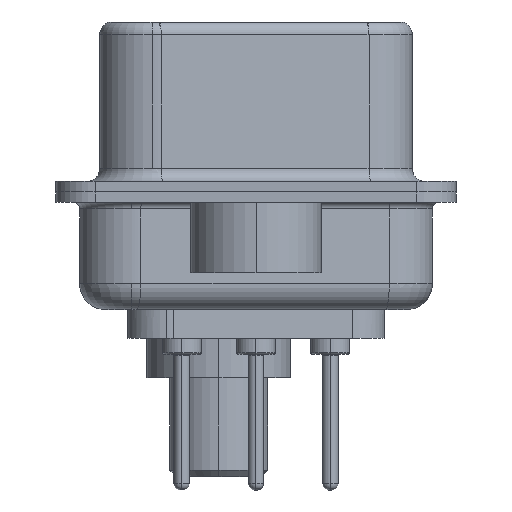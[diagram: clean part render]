
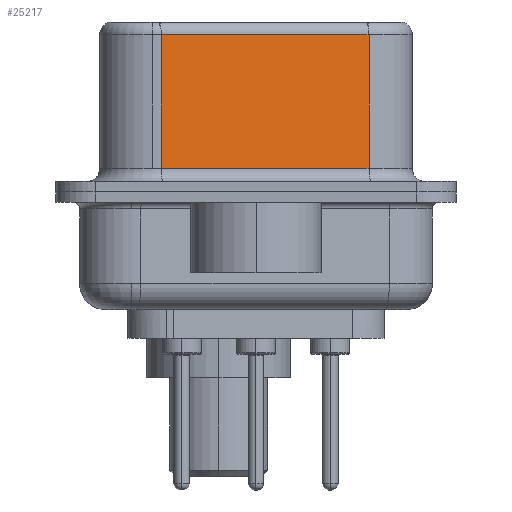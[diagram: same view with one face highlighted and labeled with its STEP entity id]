
A CAD part, left-side view. The second image highlights one B-rep face of the part: STEP entity #25217.
In plain terms, the highlighted planar face has unit normal (-0.985, -0.174, 0).
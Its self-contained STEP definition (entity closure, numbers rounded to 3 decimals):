
#1326 = AXIS2_PLACEMENT_3D ( 'NONE', #9532, #11748, #26969 ) ;
#1716 = VERTEX_POINT ( 'NONE', #25564 ) ;
#1884 = CARTESIAN_POINT ( 'NONE',  ( 3.73, 3.628, 6.52 ) ) ;
#2103 = EDGE_CURVE ( 'NONE', #10465, #1716, #22471, .T. ) ;
#4481 = CARTESIAN_POINT ( 'NONE',  ( 5.132, -4.322, 0.9 ) ) ;
#7355 = PLANE ( 'NONE',  #1326 ) ;
#7525 = LINE ( 'NONE', #1884, #24196 ) ;
#8537 = EDGE_CURVE ( 'NONE', #21673, #17644, #7525, .T. ) ;
#9532 = CARTESIAN_POINT ( 'NONE',  ( 5.132, -4.322, 6.52 ) ) ;
#10465 = VERTEX_POINT ( 'NONE', #26105 ) ;
#10806 = DIRECTION ( 'NONE',  ( 0., 0., -1. ) ) ;
#11016 = DIRECTION ( 'NONE',  ( 0.174, -0.985, 0. ) ) ;
#11748 = DIRECTION ( 'NONE',  ( 0.985, 0.174, 0. ) ) ;
#12886 = ORIENTED_EDGE ( 'NONE', *, *, #16227, .T. ) ;
#13771 = LINE ( 'NONE', #4481, #16933 ) ;
#14318 = CARTESIAN_POINT ( 'NONE',  ( 5.132, -4.322, 6.02 ) ) ;
#14321 = CARTESIAN_POINT ( 'NONE',  ( 5.132, -4.322, 6.52 ) ) ;
#15447 = DIRECTION ( 'NONE',  ( 0., 0., -1. ) ) ;
#16227 = EDGE_CURVE ( 'NONE', #17644, #1716, #13771, .T. ) ;
#16933 = VECTOR ( 'NONE', #11016, 1000. ) ;
#17644 = VERTEX_POINT ( 'NONE', #19032 ) ;
#18451 = CARTESIAN_POINT ( 'NONE',  ( 3.73, 3.628, 6.02 ) ) ;
#19032 = CARTESIAN_POINT ( 'NONE',  ( 3.73, 3.628, 0.9 ) ) ;
#21041 = FACE_OUTER_BOUND ( 'NONE', #21581, .T. ) ;
#21581 = EDGE_LOOP ( 'NONE', ( #26382, #26264, #22708, #12886 ) ) ;
#21673 = VERTEX_POINT ( 'NONE', #18451 ) ;
#21787 = VECTOR ( 'NONE', #15447, 1000. ) ;
#22471 = LINE ( 'NONE', #14321, #21787 ) ;
#22708 = ORIENTED_EDGE ( 'NONE', *, *, #8537, .T. ) ;
#24133 = EDGE_CURVE ( 'NONE', #10465, #21673, #27572, .T. ) ;
#24196 = VECTOR ( 'NONE', #10806, 1000. ) ;
#25217 = ADVANCED_FACE ( 'NONE', ( #21041 ), #7355, .F. ) ;
#25564 = CARTESIAN_POINT ( 'NONE',  ( 5.132, -4.322, 0.9 ) ) ;
#26105 = CARTESIAN_POINT ( 'NONE',  ( 5.132, -4.322, 6.02 ) ) ;
#26215 = VECTOR ( 'NONE', #27349, 1000. ) ;
#26264 = ORIENTED_EDGE ( 'NONE', *, *, #24133, .T. ) ;
#26382 = ORIENTED_EDGE ( 'NONE', *, *, #2103, .F. ) ;
#26969 = DIRECTION ( 'NONE',  ( -0.174, 0.985, 0. ) ) ;
#27349 = DIRECTION ( 'NONE',  ( -0.174, 0.985, 0. ) ) ;
#27572 = LINE ( 'NONE', #14318, #26215 ) ;
